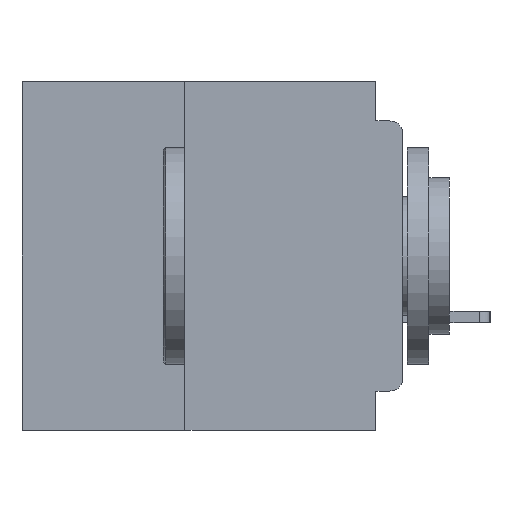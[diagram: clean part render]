
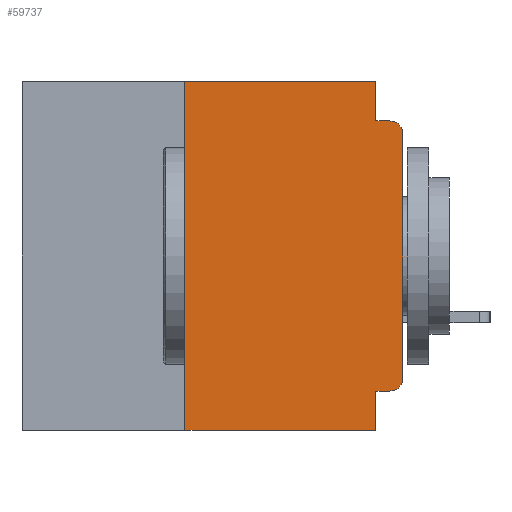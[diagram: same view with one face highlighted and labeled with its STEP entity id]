
A CAD part, left-side view. The second image highlights one B-rep face of the part: STEP entity #59737.
In plain terms, the highlighted planar face has unit normal (-1, 0, 0).
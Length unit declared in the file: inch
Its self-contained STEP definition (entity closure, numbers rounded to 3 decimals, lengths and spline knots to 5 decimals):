
#2277 = EDGE_CURVE ( 'NONE', #41921, #14402, #33067, .T. ) ;
#2343 = DIRECTION ( 'NONE',  ( 0., 0., -1. ) ) ;
#2741 = ORIENTED_EDGE ( 'NONE', *, *, #38423, .T. ) ;
#3164 = CARTESIAN_POINT ( 'NONE',  ( 0., 0., 0. ) ) ;
#3180 = CARTESIAN_POINT ( 'NONE',  ( 0., 0.25, -0.4 ) ) ;
#3354 = ORIENTED_EDGE ( 'NONE', *, *, #33814, .F. ) ;
#4126 = DIRECTION ( 'NONE',  ( 0., 0., 1. ) ) ;
#6474 = LINE ( 'NONE', #35612, #58171 ) ;
#6853 = VERTEX_POINT ( 'NONE', #58753 ) ;
#8112 = DIRECTION ( 'NONE',  ( 0., 0., 1. ) ) ;
#8748 = CARTESIAN_POINT ( 'NONE',  ( 0., 0.437, -0.4 ) ) ;
#12253 = ORIENTED_EDGE ( 'NONE', *, *, #57350, .T. ) ;
#14402 = VERTEX_POINT ( 'NONE', #51362 ) ;
#15171 = EDGE_CURVE ( 'NONE', #43981, #21828, #34220, .T. ) ;
#15320 = CARTESIAN_POINT ( 'NONE',  ( 0., 0.25, 0. ) ) ;
#15660 = ORIENTED_EDGE ( 'NONE', *, *, #40456, .F. ) ;
#15987 = VERTEX_POINT ( 'NONE', #44139 ) ;
#16226 = DIRECTION ( 'NONE',  ( -1., 0., 0. ) ) ;
#16862 = ORIENTED_EDGE ( 'NONE', *, *, #15171, .F. ) ;
#17132 = ORIENTED_EDGE ( 'NONE', *, *, #44611, .F. ) ;
#17479 = VERTEX_POINT ( 'NONE', #34327 ) ;
#18172 = CARTESIAN_POINT ( 'NONE',  ( 0., 0., -0.045 ) ) ;
#19733 = CARTESIAN_POINT ( 'NONE',  ( 0., 0.031, 0. ) ) ;
#19941 = DIRECTION ( 'NONE',  ( 0., 0., -1. ) ) ;
#20203 = VECTOR ( 'NONE', #52498, 39.37008 ) ;
#21828 = VERTEX_POINT ( 'NONE', #42908 ) ;
#22812 = CARTESIAN_POINT ( 'NONE',  ( 0., 0.031, -0.4 ) ) ;
#23329 = VECTOR ( 'NONE', #8112, 39.37008 ) ;
#23665 = AXIS2_PLACEMENT_3D ( 'NONE', #45286, #16226, #50165 ) ;
#24472 = DIRECTION ( 'NONE',  ( 0., -1., 0. ) ) ;
#26501 = VECTOR ( 'NONE', #4126, 39.37008 ) ;
#26584 = CARTESIAN_POINT ( 'NONE',  ( 0., 0.437, 0. ) ) ;
#26714 = CIRCLE ( 'NONE', #23665, 0.015 ) ;
#27263 = CARTESIAN_POINT ( 'NONE',  ( 0., 0.015, -0.355 ) ) ;
#27746 = EDGE_CURVE ( 'NONE', #56298, #14402, #43093, .T. ) ;
#28783 = EDGE_CURVE ( 'NONE', #54136, #56298, #6474, .T. ) ;
#31444 = DIRECTION ( 'NONE',  ( 0., 0., -1. ) ) ;
#31488 = DIRECTION ( 'NONE',  ( -1., 0., 0. ) ) ;
#33067 = LINE ( 'NONE', #8748, #20203 ) ;
#33814 = EDGE_CURVE ( 'NONE', #41921, #53214, #39383, .T. ) ;
#34220 = LINE ( 'NONE', #18172, #45654 ) ;
#34327 = CARTESIAN_POINT ( 'NONE',  ( 0., 0.031, 0. ) ) ;
#34811 = EDGE_CURVE ( 'NONE', #15987, #6853, #62068, .T. ) ;
#35421 = CIRCLE ( 'NONE', #47511, 0.015 ) ;
#35612 = CARTESIAN_POINT ( 'NONE',  ( 0., 0., -0.355 ) ) ;
#35709 = VECTOR ( 'NONE', #19941, 39.37008 ) ;
#36902 = ORIENTED_EDGE ( 'NONE', *, *, #2277, .T. ) ;
#37016 = FACE_OUTER_BOUND ( 'NONE', #56787, .T. ) ;
#38158 = VECTOR ( 'NONE', #24472, 39.37008 ) ;
#38423 = EDGE_CURVE ( 'NONE', #6853, #21828, #35421, .T. ) ;
#39383 = LINE ( 'NONE', #43008, #26501 ) ;
#40275 = DIRECTION ( 'NONE',  ( 0., 1., 0. ) ) ;
#40456 = EDGE_CURVE ( 'NONE', #53214, #17479, #51113, .T. ) ;
#41921 = VERTEX_POINT ( 'NONE', #3180 ) ;
#42908 = CARTESIAN_POINT ( 'NONE',  ( 0., 0.015, -0.045 ) ) ;
#43008 = CARTESIAN_POINT ( 'NONE',  ( 0., 0.25, -0.4 ) ) ;
#43093 = LINE ( 'NONE', #22812, #56039 ) ;
#43505 = CARTESIAN_POINT ( 'NONE',  ( 0., 0.031, -0.045 ) ) ;
#43981 = VERTEX_POINT ( 'NONE', #43505 ) ;
#44139 = CARTESIAN_POINT ( 'NONE',  ( 0., 0., -0.34 ) ) ;
#44611 = EDGE_CURVE ( 'NONE', #17479, #43981, #48635, .T. ) ;
#45286 = CARTESIAN_POINT ( 'NONE',  ( 0., 0.015, -0.34 ) ) ;
#45654 = VECTOR ( 'NONE', #56985, 39.37008 ) ;
#45928 = PLANE ( 'NONE',  #46555 ) ;
#46555 = AXIS2_PLACEMENT_3D ( 'NONE', #26584, #60551, #31444 ) ;
#46905 = CARTESIAN_POINT ( 'NONE',  ( 0., 0.031, -0.355 ) ) ;
#47511 = AXIS2_PLACEMENT_3D ( 'NONE', #60584, #31488, #2343 ) ;
#47584 = ORIENTED_EDGE ( 'NONE', *, *, #27746, .F. ) ;
#48635 = LINE ( 'NONE', #19733, #35709 ) ;
#49781 = ORIENTED_EDGE ( 'NONE', *, *, #28783, .F. ) ;
#50165 = DIRECTION ( 'NONE',  ( 0., 0., -1. ) ) ;
#51113 = LINE ( 'NONE', #53584, #38158 ) ;
#51362 = CARTESIAN_POINT ( 'NONE',  ( 0., 0.031, -0.4 ) ) ;
#52498 = DIRECTION ( 'NONE',  ( 0., -1., 0. ) ) ;
#53214 = VERTEX_POINT ( 'NONE', #15320 ) ;
#53584 = CARTESIAN_POINT ( 'NONE',  ( 0., 0.437, 0. ) ) ;
#54136 = VERTEX_POINT ( 'NONE', #27263 ) ;
#56039 = VECTOR ( 'NONE', #61662, 39.37008 ) ;
#56298 = VERTEX_POINT ( 'NONE', #46905 ) ;
#56787 = EDGE_LOOP ( 'NONE', ( #58569, #2741, #16862, #17132, #15660, #3354, #36902, #47584, #49781, #12253 ) ) ;
#56985 = DIRECTION ( 'NONE',  ( 0., -1., 0. ) ) ;
#57350 = EDGE_CURVE ( 'NONE', #54136, #15987, #26714, .T. ) ;
#58171 = VECTOR ( 'NONE', #40275, 39.37008 ) ;
#58569 = ORIENTED_EDGE ( 'NONE', *, *, #34811, .T. ) ;
#58753 = CARTESIAN_POINT ( 'NONE',  ( 0., 0., -0.06 ) ) ;
#59737 = ADVANCED_FACE ( 'NONE', ( #37016 ), #45928, .F. ) ;
#60551 = DIRECTION ( 'NONE',  ( 1., 0., 0. ) ) ;
#60584 = CARTESIAN_POINT ( 'NONE',  ( 0., 0.015, -0.06 ) ) ;
#61662 = DIRECTION ( 'NONE',  ( 0., 0., -1. ) ) ;
#62068 = LINE ( 'NONE', #3164, #23329 ) ;
